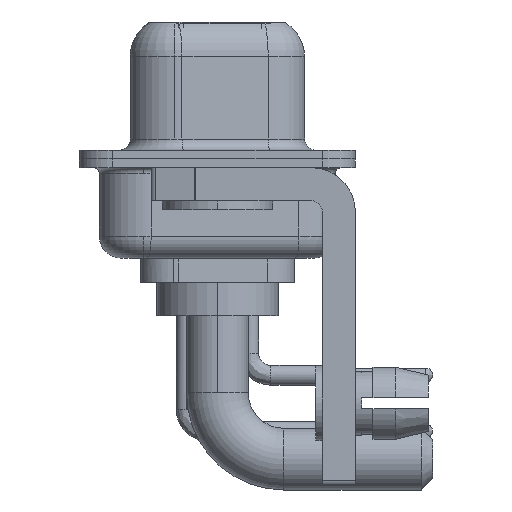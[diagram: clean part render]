
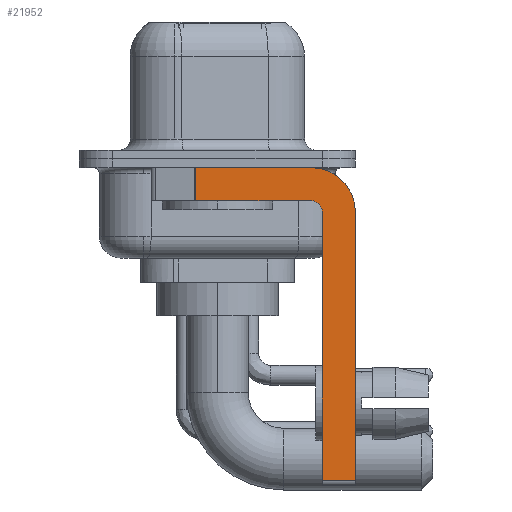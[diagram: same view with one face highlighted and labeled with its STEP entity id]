
A CAD part, left-side view. The second image highlights one B-rep face of the part: STEP entity #21952.
In plain terms, the highlighted planar face has unit normal (-1, 0, 0).
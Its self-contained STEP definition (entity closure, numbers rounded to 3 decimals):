
#24 = EDGE_LOOP ( 'NONE', ( #10668, #5375, #9078, #24639, #21062, #4130, #21930, #21201 ) ) ;
#89 = DIRECTION ( 'NONE',  ( 0., 1., 0. ) ) ;
#818 = LINE ( 'NONE', #7030, #13430 ) ;
#1346 = CARTESIAN_POINT ( 'NONE',  ( -2.9, 0.978, -1.9 ) ) ;
#2163 = VECTOR ( 'NONE', #23810, 1000. ) ;
#2326 = VERTEX_POINT ( 'NONE', #12066 ) ;
#3467 = CIRCLE ( 'NONE', #25472, 2. ) ;
#3708 = CARTESIAN_POINT ( 'NONE',  ( -2.9, 0.978, -1.9 ) ) ;
#4130 = ORIENTED_EDGE ( 'NONE', *, *, #11015, .T. ) ;
#4188 = AXIS2_PLACEMENT_3D ( 'NONE', #9221, #9491, #4960 ) ;
#4695 = CARTESIAN_POINT ( 'NONE',  ( -2.9, -6.25, -2.4 ) ) ;
#4960 = DIRECTION ( 'NONE',  ( 0., 0., -1. ) ) ;
#5375 = ORIENTED_EDGE ( 'NONE', *, *, #17103, .T. ) ;
#6093 = DIRECTION ( 'NONE',  ( 1., 0., 0. ) ) ;
#7030 = CARTESIAN_POINT ( 'NONE',  ( -2.9, 3., -0.4 ) ) ;
#8635 = DIRECTION ( 'NONE',  ( 0., 0., 1. ) ) ;
#9011 = EDGE_CURVE ( 'NONE', #19402, #26717, #3467, .T. ) ;
#9078 = ORIENTED_EDGE ( 'NONE', *, *, #24142, .F. ) ;
#9094 = FACE_OUTER_BOUND ( 'NONE', #24, .T. ) ;
#9221 = CARTESIAN_POINT ( 'NONE',  ( -2.9, -4.25, -2.4 ) ) ;
#9434 = CARTESIAN_POINT ( 'NONE',  ( -2.9, -4.25, -14.55 ) ) ;
#9491 = DIRECTION ( 'NONE',  ( 1., 0., 0. ) ) ;
#10349 = CARTESIAN_POINT ( 'NONE',  ( -2.9, -4.25, -2.4 ) ) ;
#10668 = ORIENTED_EDGE ( 'NONE', *, *, #21950, .F. ) ;
#10847 = DIRECTION ( 'NONE',  ( 0., 0., 1. ) ) ;
#11015 = EDGE_CURVE ( 'NONE', #26523, #12330, #21963, .T. ) ;
#11059 = CARTESIAN_POINT ( 'NONE',  ( -2.9, -4.75, -2.4 ) ) ;
#11931 = VECTOR ( 'NONE', #12121, 1000. ) ;
#12066 = CARTESIAN_POINT ( 'NONE',  ( -2.9, 0.978, -0.4 ) ) ;
#12121 = DIRECTION ( 'NONE',  ( 0., 0., -1. ) ) ;
#12330 = VERTEX_POINT ( 'NONE', #13309 ) ;
#13309 = CARTESIAN_POINT ( 'NONE',  ( -2.9, -6.25, -14.55 ) ) ;
#13430 = VECTOR ( 'NONE', #15143, 1000. ) ;
#13622 = EDGE_CURVE ( 'NONE', #26717, #12330, #25611, .T. ) ;
#14480 = DIRECTION ( 'NONE',  ( 0., 0., -1. ) ) ;
#14542 = CARTESIAN_POINT ( 'NONE',  ( -2.9, -4.25, -1.9 ) ) ;
#14834 = CARTESIAN_POINT ( 'NONE',  ( -2.9, -4.25, -2.4 ) ) ;
#15026 = VECTOR ( 'NONE', #8635, 1000. ) ;
#15143 = DIRECTION ( 'NONE',  ( 0., -1., 0. ) ) ;
#17103 = EDGE_CURVE ( 'NONE', #2326, #23553, #22712, .T. ) ;
#18275 = CIRCLE ( 'NONE', #18732, 0.5 ) ;
#18543 = VERTEX_POINT ( 'NONE', #18606 ) ;
#18606 = CARTESIAN_POINT ( 'NONE',  ( -2.9, -4.25, -1.9 ) ) ;
#18732 = AXIS2_PLACEMENT_3D ( 'NONE', #14834, #21564, #10847 ) ;
#18807 = CARTESIAN_POINT ( 'NONE',  ( -2.9, -4.75, -14.8 ) ) ;
#18942 = LINE ( 'NONE', #18807, #15026 ) ;
#19075 = LINE ( 'NONE', #14542, #22052 ) ;
#19402 = VERTEX_POINT ( 'NONE', #23186 ) ;
#19783 = VECTOR ( 'NONE', #24157, 1000. ) ;
#19938 = PLANE ( 'NONE',  #4188 ) ;
#20970 = EDGE_CURVE ( 'NONE', #22805, #18543, #18275, .T. ) ;
#21062 = ORIENTED_EDGE ( 'NONE', *, *, #24237, .F. ) ;
#21201 = ORIENTED_EDGE ( 'NONE', *, *, #9011, .F. ) ;
#21564 = DIRECTION ( 'NONE',  ( -1., 0., 0. ) ) ;
#21930 = ORIENTED_EDGE ( 'NONE', *, *, #13622, .F. ) ;
#21950 = EDGE_CURVE ( 'NONE', #2326, #19402, #818, .T. ) ;
#21952 = ADVANCED_FACE ( 'NONE', ( #9094 ), #19938, .F. ) ;
#21963 = LINE ( 'NONE', #9434, #19783 ) ;
#22052 = VECTOR ( 'NONE', #89, 1000. ) ;
#22712 = LINE ( 'NONE', #3708, #11931 ) ;
#22805 = VERTEX_POINT ( 'NONE', #11059 ) ;
#23186 = CARTESIAN_POINT ( 'NONE',  ( -2.9, -4.25, -0.4 ) ) ;
#23461 = CARTESIAN_POINT ( 'NONE',  ( -2.9, -6.25, -2.4 ) ) ;
#23553 = VERTEX_POINT ( 'NONE', #1346 ) ;
#23810 = DIRECTION ( 'NONE',  ( 0., 0., -1. ) ) ;
#24142 = EDGE_CURVE ( 'NONE', #18543, #23553, #19075, .T. ) ;
#24157 = DIRECTION ( 'NONE',  ( 0., -1., 0. ) ) ;
#24237 = EDGE_CURVE ( 'NONE', #26523, #22805, #18942, .T. ) ;
#24639 = ORIENTED_EDGE ( 'NONE', *, *, #20970, .F. ) ;
#25267 = CARTESIAN_POINT ( 'NONE',  ( -2.9, -4.75, -14.55 ) ) ;
#25472 = AXIS2_PLACEMENT_3D ( 'NONE', #10349, #6093, #14480 ) ;
#25611 = LINE ( 'NONE', #4695, #2163 ) ;
#26523 = VERTEX_POINT ( 'NONE', #25267 ) ;
#26717 = VERTEX_POINT ( 'NONE', #23461 ) ;
